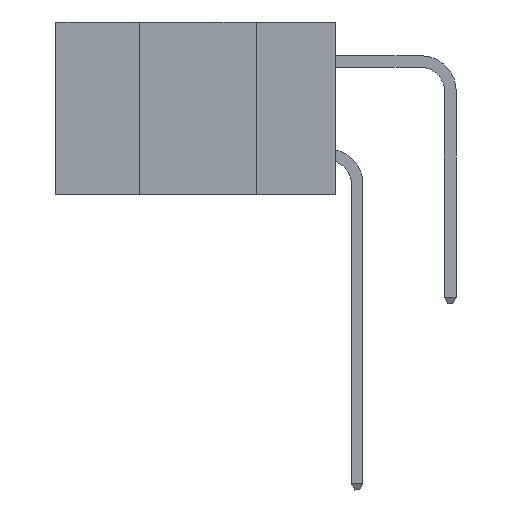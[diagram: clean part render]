
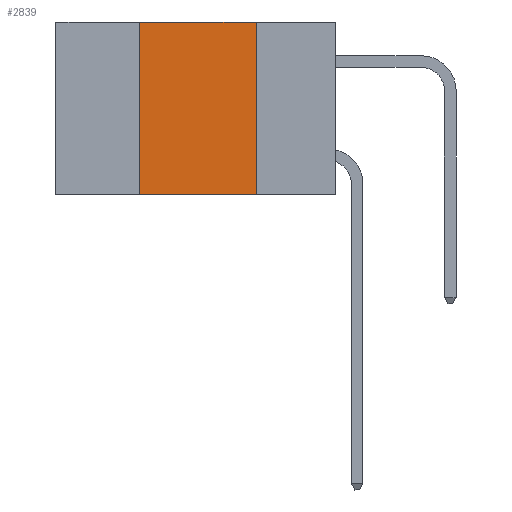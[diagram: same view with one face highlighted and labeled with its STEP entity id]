
A CAD part, left-side view. The second image highlights one B-rep face of the part: STEP entity #2839.
In plain terms, the highlighted planar face has unit normal (-1, 0, 0).
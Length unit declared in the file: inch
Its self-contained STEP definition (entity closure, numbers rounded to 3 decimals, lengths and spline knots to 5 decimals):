
#626 = LINE ( 'NONE', #2778, #11803 ) ;
#934 = ORIENTED_EDGE ( 'NONE', *, *, #12975, .F. ) ;
#1784 = VECTOR ( 'NONE', #18496, 39.37008 ) ;
#2227 = EDGE_CURVE ( 'NONE', #17738, #2701, #6704, .T. ) ;
#2701 = VERTEX_POINT ( 'NONE', #26773 ) ;
#2778 = CARTESIAN_POINT ( 'NONE',  ( 0., 0.17, 0. ) ) ;
#2839 = ADVANCED_FACE ( 'NONE', ( #8443 ), #14107, .F. ) ;
#2847 = AXIS2_PLACEMENT_3D ( 'NONE', #22694, #27362, #21054 ) ;
#3358 = CARTESIAN_POINT ( 'NONE',  ( 0., 0.42, 0. ) ) ;
#3367 = ORIENTED_EDGE ( 'NONE', *, *, #26599, .F. ) ;
#6704 = LINE ( 'NONE', #16776, #8779 ) ;
#7392 = LINE ( 'NONE', #20618, #1784 ) ;
#7790 = CARTESIAN_POINT ( 'NONE',  ( 0., 0.42, 0. ) ) ;
#8443 = FACE_OUTER_BOUND ( 'NONE', #15847, .T. ) ;
#8779 = VECTOR ( 'NONE', #23046, 39.37008 ) ;
#9065 = VERTEX_POINT ( 'NONE', #24703 ) ;
#11381 = ORIENTED_EDGE ( 'NONE', *, *, #2227, .T. ) ;
#11803 = VECTOR ( 'NONE', #27850, 39.37008 ) ;
#12234 = CARTESIAN_POINT ( 'NONE',  ( 0., 0.42, -0.37 ) ) ;
#12975 = EDGE_CURVE ( 'NONE', #9065, #2701, #626, .T. ) ;
#13085 = EDGE_CURVE ( 'NONE', #17738, #25765, #17721, .T. ) ;
#14107 = PLANE ( 'NONE',  #2847 ) ;
#15847 = EDGE_LOOP ( 'NONE', ( #934, #3367, #25133, #11381 ) ) ;
#16698 = VECTOR ( 'NONE', #25790, 39.37008 ) ;
#16776 = CARTESIAN_POINT ( 'NONE',  ( 0., 0.6, -0.37 ) ) ;
#17721 = LINE ( 'NONE', #3358, #16698 ) ;
#17738 = VERTEX_POINT ( 'NONE', #12234 ) ;
#18496 = DIRECTION ( 'NONE',  ( 0., -1., 0. ) ) ;
#20618 = CARTESIAN_POINT ( 'NONE',  ( 0., 0.6, 0. ) ) ;
#21054 = DIRECTION ( 'NONE',  ( 0., 0., -1. ) ) ;
#22694 = CARTESIAN_POINT ( 'NONE',  ( 0., 0.6, 0. ) ) ;
#23046 = DIRECTION ( 'NONE',  ( 0., -1., 0. ) ) ;
#24703 = CARTESIAN_POINT ( 'NONE',  ( 0., 0.17, 0. ) ) ;
#25133 = ORIENTED_EDGE ( 'NONE', *, *, #13085, .F. ) ;
#25765 = VERTEX_POINT ( 'NONE', #7790 ) ;
#25790 = DIRECTION ( 'NONE',  ( 0., 0., 1. ) ) ;
#26599 = EDGE_CURVE ( 'NONE', #25765, #9065, #7392, .T. ) ;
#26773 = CARTESIAN_POINT ( 'NONE',  ( 0., 0.17, -0.37 ) ) ;
#27362 = DIRECTION ( 'NONE',  ( 1., 0., 0. ) ) ;
#27850 = DIRECTION ( 'NONE',  ( 0., 0., -1. ) ) ;
